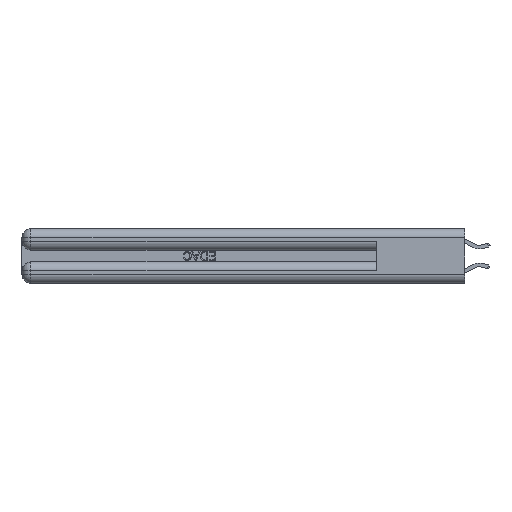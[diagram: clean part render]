
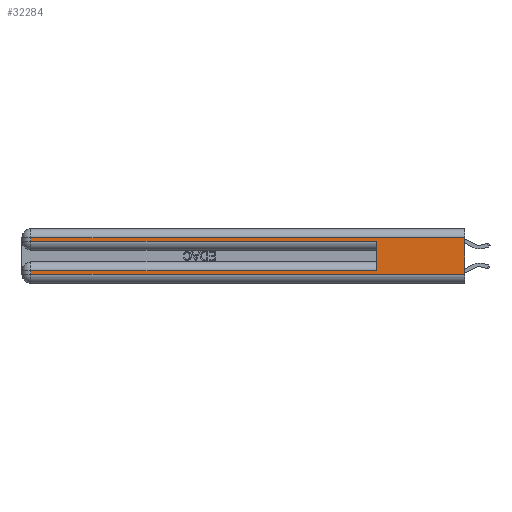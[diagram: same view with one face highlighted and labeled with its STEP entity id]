
A CAD part, left-side view. The second image highlights one B-rep face of the part: STEP entity #32284.
In plain terms, the highlighted planar face has unit normal (-1, 0, 0).
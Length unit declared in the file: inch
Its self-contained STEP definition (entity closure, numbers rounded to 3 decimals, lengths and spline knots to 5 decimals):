
#539 = DIRECTION ( 'NONE',  ( 0., 0., -1. ) ) ;
#855 = VECTOR ( 'NONE', #7148, 39.37008 ) ;
#1227 = VECTOR ( 'NONE', #1700, 39.37008 ) ;
#1700 = DIRECTION ( 'NONE',  ( 0., 1., 0. ) ) ;
#1907 = VECTOR ( 'NONE', #33569, 39.37008 ) ;
#3048 = VECTOR ( 'NONE', #22144, 39.37008 ) ;
#3075 = CARTESIAN_POINT ( 'NONE',  ( 0., 2.94, 0.06 ) ) ;
#3388 = LINE ( 'NONE', #26377, #34220 ) ;
#5558 = ORIENTED_EDGE ( 'NONE', *, *, #9819, .F. ) ;
#6204 = DIRECTION ( 'NONE',  ( 0., 0., -1. ) ) ;
#7036 = ORIENTED_EDGE ( 'NONE', *, *, #32632, .F. ) ;
#7148 = DIRECTION ( 'NONE',  ( 0., -1., 0. ) ) ;
#7178 = DIRECTION ( 'NONE',  ( 1., 0., 0. ) ) ;
#9819 = EDGE_CURVE ( 'NONE', #31159, #14343, #3388, .T. ) ;
#13211 = DIRECTION ( 'NONE',  ( 0., 0., -1. ) ) ;
#13360 = AXIS2_PLACEMENT_3D ( 'NONE', #31930, #7178, #34443 ) ;
#14343 = VERTEX_POINT ( 'NONE', #33832 ) ;
#15078 = EDGE_CURVE ( 'NONE', #23271, #22036, #27891, .T. ) ;
#15426 = LINE ( 'NONE', #23854, #855 ) ;
#15947 = VECTOR ( 'NONE', #6204, 39.37008 ) ;
#16079 = CARTESIAN_POINT ( 'NONE',  ( 0., 2.94, 0.285 ) ) ;
#17723 = LINE ( 'NONE', #31150, #1907 ) ;
#17915 = LINE ( 'NONE', #18073, #1227 ) ;
#18073 = CARTESIAN_POINT ( 'NONE',  ( 0., 0., 0.085 ) ) ;
#19442 = CARTESIAN_POINT ( 'NONE',  ( 0., 0.6, 0.085 ) ) ;
#19788 = ORIENTED_EDGE ( 'NONE', *, *, #15078, .T. ) ;
#19802 = CARTESIAN_POINT ( 'NONE',  ( 0., 0., 0.37 ) ) ;
#20052 = EDGE_CURVE ( 'NONE', #25571, #34558, #28675, .T. ) ;
#20298 = CARTESIAN_POINT ( 'NONE',  ( 0., 2.94, 0.37 ) ) ;
#21011 = CARTESIAN_POINT ( 'NONE',  ( 0., 0., 0.06 ) ) ;
#21181 = VERTEX_POINT ( 'NONE', #21011 ) ;
#21415 = VECTOR ( 'NONE', #13211, 39.37008 ) ;
#21781 = FACE_OUTER_BOUND ( 'NONE', #31291, .T. ) ;
#22036 = VERTEX_POINT ( 'NONE', #30823 ) ;
#22144 = DIRECTION ( 'NONE',  ( 0., 1., 0. ) ) ;
#23177 = ORIENTED_EDGE ( 'NONE', *, *, #23911, .T. ) ;
#23194 = LINE ( 'NONE', #20298, #15947 ) ;
#23271 = VERTEX_POINT ( 'NONE', #24418 ) ;
#23835 = LINE ( 'NONE', #19802, #28160 ) ;
#23854 = CARTESIAN_POINT ( 'NONE',  ( 0., 0., 0.06 ) ) ;
#23911 = EDGE_CURVE ( 'NONE', #34558, #21181, #15426, .T. ) ;
#24076 = DIRECTION ( 'NONE',  ( 0., 0., 1. ) ) ;
#24418 = CARTESIAN_POINT ( 'NONE',  ( 0., 0., 0.31 ) ) ;
#25005 = CARTESIAN_POINT ( 'NONE',  ( 0., 2.94, 0.085 ) ) ;
#25241 = CARTESIAN_POINT ( 'NONE',  ( 0., 0., 0.31 ) ) ;
#25510 = VERTEX_POINT ( 'NONE', #16079 ) ;
#25571 = VERTEX_POINT ( 'NONE', #25005 ) ;
#26025 = ORIENTED_EDGE ( 'NONE', *, *, #20052, .T. ) ;
#26058 = PLANE ( 'NONE',  #13360 ) ;
#26377 = CARTESIAN_POINT ( 'NONE',  ( 0., 0.6, 0.145 ) ) ;
#27891 = LINE ( 'NONE', #25241, #3048 ) ;
#28160 = VECTOR ( 'NONE', #539, 39.37008 ) ;
#28194 = EDGE_CURVE ( 'NONE', #25510, #14343, #17723, .T. ) ;
#28378 = ORIENTED_EDGE ( 'NONE', *, *, #29300, .T. ) ;
#28675 = LINE ( 'NONE', #29809, #21415 ) ;
#29300 = EDGE_CURVE ( 'NONE', #22036, #25510, #23194, .T. ) ;
#29809 = CARTESIAN_POINT ( 'NONE',  ( 0., 2.94, 0.37 ) ) ;
#30823 = CARTESIAN_POINT ( 'NONE',  ( 0., 2.94, 0.31 ) ) ;
#31150 = CARTESIAN_POINT ( 'NONE',  ( 0., 0., 0.285 ) ) ;
#31159 = VERTEX_POINT ( 'NONE', #19442 ) ;
#31291 = EDGE_LOOP ( 'NONE', ( #7036, #19788, #28378, #34641, #5558, #33355, #26025, #23177 ) ) ;
#31739 = EDGE_CURVE ( 'NONE', #31159, #25571, #17915, .T. ) ;
#31930 = CARTESIAN_POINT ( 'NONE',  ( 0., 0., 0.37 ) ) ;
#32284 = ADVANCED_FACE ( 'NONE', ( #21781 ), #26058, .F. ) ;
#32632 = EDGE_CURVE ( 'NONE', #23271, #21181, #23835, .T. ) ;
#33355 = ORIENTED_EDGE ( 'NONE', *, *, #31739, .T. ) ;
#33569 = DIRECTION ( 'NONE',  ( 0., -1., 0. ) ) ;
#33832 = CARTESIAN_POINT ( 'NONE',  ( 0., 0.6, 0.285 ) ) ;
#34220 = VECTOR ( 'NONE', #24076, 39.37008 ) ;
#34443 = DIRECTION ( 'NONE',  ( 0., 0., -1. ) ) ;
#34558 = VERTEX_POINT ( 'NONE', #3075 ) ;
#34641 = ORIENTED_EDGE ( 'NONE', *, *, #28194, .T. ) ;
